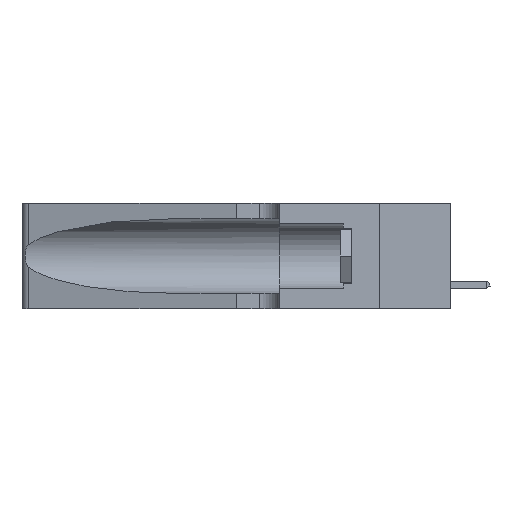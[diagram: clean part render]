
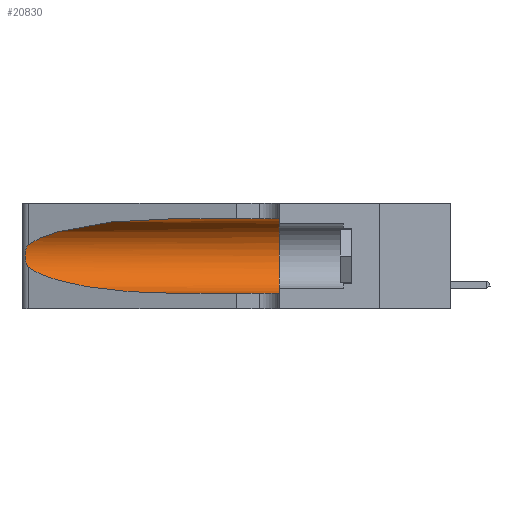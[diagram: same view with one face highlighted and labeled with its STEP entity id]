
A CAD part, left-side view. The second image highlights one B-rep face of the part: STEP entity #20830.
In plain terms, the highlighted cylindrical face has radius 3.308 mm (diameter 6.617 mm), a partial arc.
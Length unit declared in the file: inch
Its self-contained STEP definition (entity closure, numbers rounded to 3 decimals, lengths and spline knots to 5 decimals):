
#225 = VERTEX_POINT ( 'NONE', #26096 ) ;
#1083 = EDGE_CURVE ( 'NONE', #4266, #19642, #15952, .T. ) ;
#1863 = DIRECTION ( 'NONE',  ( 0., -1., 0. ) ) ;
#2438 = CARTESIAN_POINT ( 'NONE',  ( 0.26075, 1.23896, 0.178 ) ) ;
#2562 = CARTESIAN_POINT ( 'NONE',  ( 0.26018, 1.23835, 0.19895 ) ) ;
#2795 = CARTESIAN_POINT ( 'NONE',  ( 0.1305, 0.35, 0.31525 ) ) ;
#3301 = CARTESIAN_POINT ( 'NONE',  ( 0.1305, 0.35, 0.185 ) ) ;
#3533 = DIRECTION ( 'NONE',  ( 0., 1., 0. ) ) ;
#3998 = DIRECTION ( 'NONE',  ( 0., -1., 0. ) ) ;
#4266 = VERTEX_POINT ( 'NONE', #23057 ) ;
#6077 = EDGE_LOOP ( 'NONE', ( #31748, #16962, #28116, #32777, #26153, #17074 ) ) ;
#8400 = EDGE_CURVE ( 'NONE', #8807, #19642, #34491, .T. ) ;
#8631 = B_SPLINE_CURVE_WITH_KNOTS ( 'NONE', 3,
 ( #35637, #13626, #27220, #13248, #29983, #2562, #19135, #2438, #27105, #27341, #26974, #21651, #10617, #10856 ),
 .UNSPECIFIED., .F., .F.,
 ( 4, 2, 2, 2, 2, 2, 4 ),
 ( 0., 0.00027, 0.00053, 0.00107, 0.0016, 0.00187, 0.00214 ),
 .UNSPECIFIED. ) ;
#8807 = VERTEX_POINT ( 'NONE', #2795 ) ;
#8940 = DIRECTION ( 'NONE',  ( 0., 0., 1. ) ) ;
#9109 = VECTOR ( 'NONE', #26074, 39.37008 ) ;
#10617 = CARTESIAN_POINT ( 'NONE',  ( 0.25555, 1.22993, 0.14849 ) ) ;
#10856 = CARTESIAN_POINT ( 'NONE',  ( 0.25487, 1.22718, 0.14631 ) ) ;
#12444 = CARTESIAN_POINT ( 'NONE',  ( 0.1305, 1.61858, 0.31525 ) ) ;
#12559 = CARTESIAN_POINT ( 'NONE',  ( 0.2373, 1.15595, 0.28018 ) ) ;
#13248 = CARTESIAN_POINT ( 'NONE',  ( 0.25787, 1.23484, 0.2124 ) ) ;
#13626 = CARTESIAN_POINT ( 'NONE',  ( 0.25555, 1.22994, 0.2215 ) ) ;
#15952 = LINE ( 'NONE', #16729, #9109 ) ;
#16026 = CYLINDRICAL_SURFACE ( 'NONE', #18011, 0.13025 ) ;
#16729 = CARTESIAN_POINT ( 'NONE',  ( 0.1305, 1.61858, 0.05475 ) ) ;
#16962 = ORIENTED_EDGE ( 'NONE', *, *, #23920, .T. ) ;
#17074 = ORIENTED_EDGE ( 'NONE', *, *, #23068, .F. ) ;
#17399 = CARTESIAN_POINT ( 'NONE',  ( 0.1305, 0.35, 0.05475 ) ) ;
#17969 = EDGE_CURVE ( 'NONE', #225, #4266, #18276, .T. ) ;
#18011 = AXIS2_PLACEMENT_3D ( 'NONE', #23202, #3998, #25005 ) ;
#18125 = CARTESIAN_POINT ( 'NONE',  ( 0.25487, 1.22718, 0.14631 ) ) ;
#18276 =( BOUNDED_CURVE ( )  B_SPLINE_CURVE ( 3, ( #18125, #29457, #32097, #31616 ),
 .UNSPECIFIED., .F., .T. ) 
 B_SPLINE_CURVE_WITH_KNOTS ( ( 4, 4 ),
 ( 3.44316, 4.71239 ),
 .UNSPECIFIED. ) 
 CURVE ( )  GEOMETRIC_REPRESENTATION_ITEM ( )  RATIONAL_B_SPLINE_CURVE ( ( 1., 0.87, 0.87, 1. ) ) 
 REPRESENTATION_ITEM ( '' )  );
#19135 = CARTESIAN_POINT ( 'NONE',  ( 0.26075, 1.23896, 0.19203 ) ) ;
#19642 = VERTEX_POINT ( 'NONE', #17399 ) ;
#19969 = CARTESIAN_POINT ( 'NONE',  ( 0.25487, 1.22718, 0.22369 ) ) ;
#20266 = CARTESIAN_POINT ( 'NONE',  ( 0.18966, 0.96281, 0.31525 ) ) ;
#20830 = ADVANCED_FACE ( 'NONE', ( #26790 ), #16026, .F. ) ;
#21651 = CARTESIAN_POINT ( 'NONE',  ( 0.25639, 1.23186, 0.15144 ) ) ;
#21666 = VERTEX_POINT ( 'NONE', #19969 ) ;
#22488 =( BOUNDED_CURVE ( )  B_SPLINE_CURVE ( 3, ( #28486, #20266, #12559, #23848 ),
 .UNSPECIFIED., .F., .F. ) 
 B_SPLINE_CURVE_WITH_KNOTS ( ( 4, 4 ),
 ( 1.5708, 2.84003 ),
 .UNSPECIFIED. ) 
 CURVE ( )  GEOMETRIC_REPRESENTATION_ITEM ( )  RATIONAL_B_SPLINE_CURVE ( ( 1., 0.87, 0.87, 1. ) ) 
 REPRESENTATION_ITEM ( '' )  );
#23020 = EDGE_CURVE ( 'NONE', #34251, #21666, #22488, .T. ) ;
#23057 = CARTESIAN_POINT ( 'NONE',  ( 0.1305, 0.72297, 0.05475 ) ) ;
#23068 = EDGE_CURVE ( 'NONE', #34251, #8807, #25809, .T. ) ;
#23202 = CARTESIAN_POINT ( 'NONE',  ( 0.1305, 1.61858, 0.185 ) ) ;
#23848 = CARTESIAN_POINT ( 'NONE',  ( 0.25487, 1.22718, 0.22369 ) ) ;
#23920 = EDGE_CURVE ( 'NONE', #21666, #225, #8631, .T. ) ;
#25005 = DIRECTION ( 'NONE',  ( 0., 0., -1. ) ) ;
#25744 = VECTOR ( 'NONE', #1863, 39.37008 ) ;
#25809 = LINE ( 'NONE', #12444, #25744 ) ;
#26074 = DIRECTION ( 'NONE',  ( 0., -1., 0. ) ) ;
#26096 = CARTESIAN_POINT ( 'NONE',  ( 0.25487, 1.22718, 0.14631 ) ) ;
#26153 = ORIENTED_EDGE ( 'NONE', *, *, #8400, .F. ) ;
#26790 = FACE_OUTER_BOUND ( 'NONE', #6077, .T. ) ;
#26974 = CARTESIAN_POINT ( 'NONE',  ( 0.25789, 1.23486, 0.15765 ) ) ;
#27105 = CARTESIAN_POINT ( 'NONE',  ( 0.26017, 1.23833, 0.17102 ) ) ;
#27220 = CARTESIAN_POINT ( 'NONE',  ( 0.25639, 1.23184, 0.21858 ) ) ;
#27341 = CARTESIAN_POINT ( 'NONE',  ( 0.25856, 1.23593, 0.16098 ) ) ;
#28116 = ORIENTED_EDGE ( 'NONE', *, *, #17969, .T. ) ;
#28486 = CARTESIAN_POINT ( 'NONE',  ( 0.1305, 0.72297, 0.31525 ) ) ;
#29102 = AXIS2_PLACEMENT_3D ( 'NONE', #3301, #3533, #8940 ) ;
#29457 = CARTESIAN_POINT ( 'NONE',  ( 0.2373, 1.15595, 0.08982 ) ) ;
#29983 = CARTESIAN_POINT ( 'NONE',  ( 0.25854, 1.2359, 0.20912 ) ) ;
#31616 = CARTESIAN_POINT ( 'NONE',  ( 0.1305, 0.72297, 0.05475 ) ) ;
#31748 = ORIENTED_EDGE ( 'NONE', *, *, #23020, .T. ) ;
#32097 = CARTESIAN_POINT ( 'NONE',  ( 0.18966, 0.96281, 0.05475 ) ) ;
#32777 = ORIENTED_EDGE ( 'NONE', *, *, #1083, .T. ) ;
#34251 = VERTEX_POINT ( 'NONE', #35242 ) ;
#34491 = CIRCLE ( 'NONE', #29102, 0.13025 ) ;
#35242 = CARTESIAN_POINT ( 'NONE',  ( 0.1305, 0.72297, 0.31525 ) ) ;
#35637 = CARTESIAN_POINT ( 'NONE',  ( 0.25487, 1.22718, 0.22369 ) ) ;
